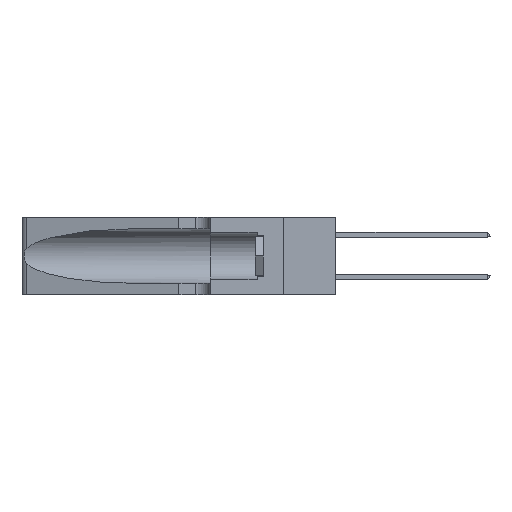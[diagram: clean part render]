
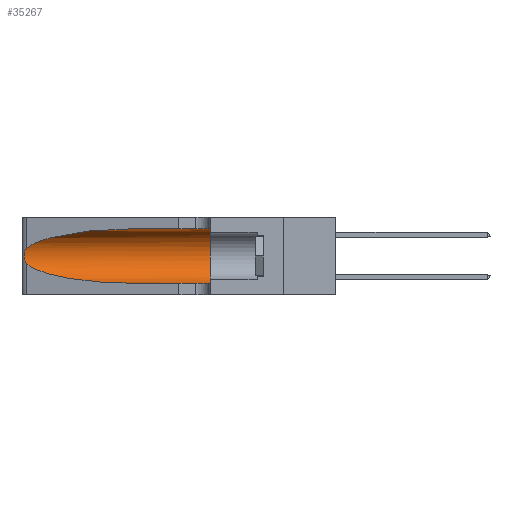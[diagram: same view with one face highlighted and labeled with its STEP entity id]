
A CAD part, left-side view. The second image highlights one B-rep face of the part: STEP entity #35267.
In plain terms, the highlighted cylindrical face has radius 3.308 mm (diameter 6.617 mm), a partial arc.
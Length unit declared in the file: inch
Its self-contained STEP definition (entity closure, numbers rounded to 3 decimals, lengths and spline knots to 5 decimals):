
#1326 = DIRECTION ( 'NONE',  ( 0., 0., 1. ) ) ;
#2000 = CARTESIAN_POINT ( 'NONE',  ( 0.25487, 1.22718, 0.22369 ) ) ;
#2438 = CARTESIAN_POINT ( 'NONE',  ( 0.25555, 1.22994, 0.2215 ) ) ;
#2598 = CARTESIAN_POINT ( 'NONE',  ( 0.25639, 1.23186, 0.15144 ) ) ;
#4272 = CYLINDRICAL_SURFACE ( 'NONE', #12269, 0.13025 ) ;
#4472 = AXIS2_PLACEMENT_3D ( 'NONE', #47485, #24680, #1326 ) ;
#5768 = CARTESIAN_POINT ( 'NONE',  ( 0.25487, 1.22718, 0.14631 ) ) ;
#6617 = CARTESIAN_POINT ( 'NONE',  ( 0.25487, 1.22718, 0.14631 ) ) ;
#7225 = ORIENTED_EDGE ( 'NONE', *, *, #40824, .T. ) ;
#9180 = ORIENTED_EDGE ( 'NONE', *, *, #9565, .F. ) ;
#9565 = EDGE_CURVE ( 'NONE', #43114, #28060, #38066, .T. ) ;
#9772 = CARTESIAN_POINT ( 'NONE',  ( 0.2373, 1.15595, 0.08982 ) ) ;
#10440 = CARTESIAN_POINT ( 'NONE',  ( 0.25639, 1.23184, 0.21858 ) ) ;
#11609 = EDGE_LOOP ( 'NONE', ( #13479, #7225, #32780, #27610, #40532, #9180 ) ) ;
#12269 = AXIS2_PLACEMENT_3D ( 'NONE', #21561, #36736, #48218 ) ;
#12781 = VERTEX_POINT ( 'NONE', #14544 ) ;
#13479 = ORIENTED_EDGE ( 'NONE', *, *, #22592, .T. ) ;
#13498 = CARTESIAN_POINT ( 'NONE',  ( 0.1305, 1.61858, 0.05475 ) ) ;
#13724 = CARTESIAN_POINT ( 'NONE',  ( 0.1305, 0.72297, 0.31525 ) ) ;
#14248 = VECTOR ( 'NONE', #17363, 39.37008 ) ;
#14304 = CARTESIAN_POINT ( 'NONE',  ( 0.25854, 1.2359, 0.20912 ) ) ;
#14488 = CARTESIAN_POINT ( 'NONE',  ( 0.1305, 0.72297, 0.05475 ) ) ;
#14544 = CARTESIAN_POINT ( 'NONE',  ( 0.25487, 1.22718, 0.14631 ) ) ;
#17115 = EDGE_CURVE ( 'NONE', #28060, #40915, #21044, .T. ) ;
#17363 = DIRECTION ( 'NONE',  ( 0., -1., 0. ) ) ;
#17447 = VERTEX_POINT ( 'NONE', #30154 ) ;
#17518 = CARTESIAN_POINT ( 'NONE',  ( 0.1305, 0.72297, 0.05475 ) ) ;
#17748 = VECTOR ( 'NONE', #45299, 39.37008 ) ;
#18182 = CARTESIAN_POINT ( 'NONE',  ( 0.26075, 1.23896, 0.19203 ) ) ;
#21044 = CIRCLE ( 'NONE', #4472, 0.13025 ) ;
#21561 = CARTESIAN_POINT ( 'NONE',  ( 0.1305, 1.61858, 0.185 ) ) ;
#22082 = CARTESIAN_POINT ( 'NONE',  ( 0.26017, 1.23833, 0.17102 ) ) ;
#22592 = EDGE_CURVE ( 'NONE', #43114, #17447, #23692, .T. ) ;
#23692 =( BOUNDED_CURVE ( )  B_SPLINE_CURVE ( 3, ( #13724, #40480, #25351, #2000 ),
 .UNSPECIFIED., .F., .F. ) 
 B_SPLINE_CURVE_WITH_KNOTS ( ( 4, 4 ),
 ( 1.5708, 2.84003 ),
 .UNSPECIFIED. ) 
 CURVE ( )  GEOMETRIC_REPRESENTATION_ITEM ( )  RATIONAL_B_SPLINE_CURVE ( ( 1., 0.87, 0.87, 1. ) ) 
 REPRESENTATION_ITEM ( '' )  );
#24680 = DIRECTION ( 'NONE',  ( 0., 1., 0. ) ) ;
#24977 = FACE_OUTER_BOUND ( 'NONE', #11609, .T. ) ;
#25351 = CARTESIAN_POINT ( 'NONE',  ( 0.2373, 1.15595, 0.28018 ) ) ;
#25913 = CARTESIAN_POINT ( 'NONE',  ( 0.25789, 1.23486, 0.15765 ) ) ;
#26404 = CARTESIAN_POINT ( 'NONE',  ( 0.1305, 0.35, 0.05475 ) ) ;
#27610 = ORIENTED_EDGE ( 'NONE', *, *, #30393, .T. ) ;
#28060 = VERTEX_POINT ( 'NONE', #38449 ) ;
#28550 = VERTEX_POINT ( 'NONE', #14488 ) ;
#28920 = B_SPLINE_CURVE_WITH_KNOTS ( 'NONE', 3,
 ( #29594, #2438, #10440, #37239, #14304, #41056, #18182, #44870, #22082, #48717, #25913, #2598, #29764, #6617 ),
 .UNSPECIFIED., .F., .F.,
 ( 4, 2, 2, 2, 2, 2, 4 ),
 ( 0., 0.00027, 0.00053, 0.00107, 0.0016, 0.00187, 0.00214 ),
 .UNSPECIFIED. ) ;
#29594 = CARTESIAN_POINT ( 'NONE',  ( 0.25487, 1.22718, 0.22369 ) ) ;
#29764 = CARTESIAN_POINT ( 'NONE',  ( 0.25555, 1.22993, 0.14849 ) ) ;
#30154 = CARTESIAN_POINT ( 'NONE',  ( 0.25487, 1.22718, 0.22369 ) ) ;
#30393 = EDGE_CURVE ( 'NONE', #28550, #40915, #44742, .T. ) ;
#32780 = ORIENTED_EDGE ( 'NONE', *, *, #40737, .T. ) ;
#35267 = ADVANCED_FACE ( 'NONE', ( #24977 ), #4272, .F. ) ;
#36736 = DIRECTION ( 'NONE',  ( 0., -1., 0. ) ) ;
#37239 = CARTESIAN_POINT ( 'NONE',  ( 0.25787, 1.23484, 0.2124 ) ) ;
#37735 =( BOUNDED_CURVE ( )  B_SPLINE_CURVE ( 3, ( #5768, #9772, #40413, #17518 ),
 .UNSPECIFIED., .F., .F. ) 
 B_SPLINE_CURVE_WITH_KNOTS ( ( 4, 4 ),
 ( 3.44316, 4.71239 ),
 .UNSPECIFIED. ) 
 CURVE ( )  GEOMETRIC_REPRESENTATION_ITEM ( )  RATIONAL_B_SPLINE_CURVE ( ( 1., 0.87, 0.87, 1. ) ) 
 REPRESENTATION_ITEM ( '' )  );
#38066 = LINE ( 'NONE', #41496, #17748 ) ;
#38449 = CARTESIAN_POINT ( 'NONE',  ( 0.1305, 0.35, 0.31525 ) ) ;
#40413 = CARTESIAN_POINT ( 'NONE',  ( 0.18966, 0.96281, 0.05475 ) ) ;
#40480 = CARTESIAN_POINT ( 'NONE',  ( 0.18966, 0.96281, 0.31525 ) ) ;
#40532 = ORIENTED_EDGE ( 'NONE', *, *, #17115, .F. ) ;
#40737 = EDGE_CURVE ( 'NONE', #12781, #28550, #37735, .T. ) ;
#40824 = EDGE_CURVE ( 'NONE', #17447, #12781, #28920, .T. ) ;
#40915 = VERTEX_POINT ( 'NONE', #26404 ) ;
#41056 = CARTESIAN_POINT ( 'NONE',  ( 0.26018, 1.23835, 0.19895 ) ) ;
#41496 = CARTESIAN_POINT ( 'NONE',  ( 0.1305, 1.61858, 0.31525 ) ) ;
#42024 = CARTESIAN_POINT ( 'NONE',  ( 0.1305, 0.72297, 0.31525 ) ) ;
#43114 = VERTEX_POINT ( 'NONE', #42024 ) ;
#44742 = LINE ( 'NONE', #13498, #14248 ) ;
#44870 = CARTESIAN_POINT ( 'NONE',  ( 0.26075, 1.23896, 0.178 ) ) ;
#45299 = DIRECTION ( 'NONE',  ( 0., -1., 0. ) ) ;
#47485 = CARTESIAN_POINT ( 'NONE',  ( 0.1305, 0.35, 0.185 ) ) ;
#48218 = DIRECTION ( 'NONE',  ( 0., 0., -1. ) ) ;
#48717 = CARTESIAN_POINT ( 'NONE',  ( 0.25856, 1.23593, 0.16098 ) ) ;
